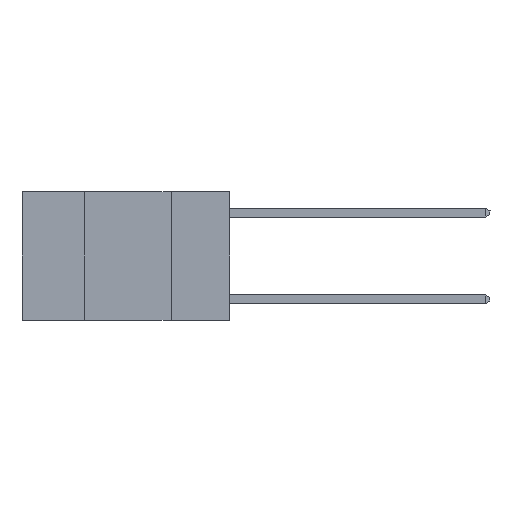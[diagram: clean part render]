
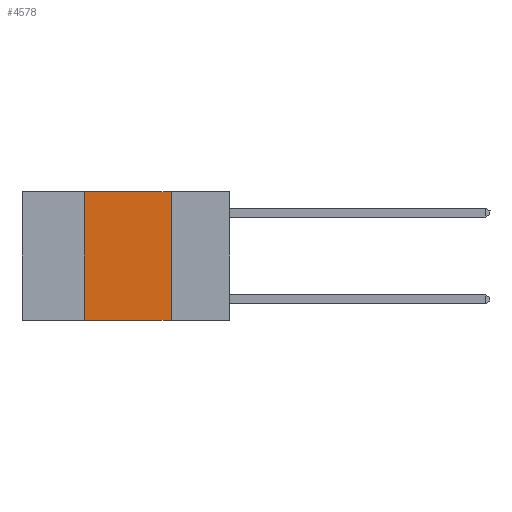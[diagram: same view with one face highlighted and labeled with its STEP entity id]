
A CAD part, left-side view. The second image highlights one B-rep face of the part: STEP entity #4578.
In plain terms, the highlighted planar face has unit normal (-1, 0, 0).
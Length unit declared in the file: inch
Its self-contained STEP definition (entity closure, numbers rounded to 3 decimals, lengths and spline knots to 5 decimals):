
#58 = VERTEX_POINT ( 'NONE', #2633 ) ;
#358 = VECTOR ( 'NONE', #4626, 39.37008 ) ;
#368 = CARTESIAN_POINT ( 'NONE',  ( 0., 0.42, -0.37 ) ) ;
#1398 = DIRECTION ( 'NONE',  ( 0., 0., 1. ) ) ;
#1654 = VECTOR ( 'NONE', #1398, 39.37008 ) ;
#1750 = EDGE_CURVE ( 'NONE', #11668, #8958, #3074, .T. ) ;
#1890 = VECTOR ( 'NONE', #10463, 39.37008 ) ;
#2633 = CARTESIAN_POINT ( 'NONE',  ( 0., 0.17, -0.37 ) ) ;
#2712 = PLANE ( 'NONE',  #10437 ) ;
#2893 = VERTEX_POINT ( 'NONE', #368 ) ;
#3074 = LINE ( 'NONE', #10550, #358 ) ;
#3284 = CARTESIAN_POINT ( 'NONE',  ( 0., 0.6, -0.37 ) ) ;
#3461 = LINE ( 'NONE', #3741, #5875 ) ;
#3641 = DIRECTION ( 'NONE',  ( 1., 0., 0. ) ) ;
#3741 = CARTESIAN_POINT ( 'NONE',  ( 0., 0.17, 0. ) ) ;
#4429 = ORIENTED_EDGE ( 'NONE', *, *, #9628, .T. ) ;
#4501 = CARTESIAN_POINT ( 'NONE',  ( 0., 0.6, 0. ) ) ;
#4578 = ADVANCED_FACE ( 'NONE', ( #8451 ), #2712, .F. ) ;
#4626 = DIRECTION ( 'NONE',  ( 0., -1., 0. ) ) ;
#5115 = CARTESIAN_POINT ( 'NONE',  ( 0., 0.17, 0. ) ) ;
#5264 = EDGE_CURVE ( 'NONE', #2893, #11668, #6473, .T. ) ;
#5408 = EDGE_LOOP ( 'NONE', ( #8092, #6256, #6558, #4429 ) ) ;
#5875 = VECTOR ( 'NONE', #10898, 39.37008 ) ;
#6256 = ORIENTED_EDGE ( 'NONE', *, *, #1750, .F. ) ;
#6473 = LINE ( 'NONE', #6831, #1654 ) ;
#6558 = ORIENTED_EDGE ( 'NONE', *, *, #5264, .F. ) ;
#6831 = CARTESIAN_POINT ( 'NONE',  ( 0., 0.42, 0. ) ) ;
#8092 = ORIENTED_EDGE ( 'NONE', *, *, #9266, .F. ) ;
#8451 = FACE_OUTER_BOUND ( 'NONE', #5408, .T. ) ;
#8958 = VERTEX_POINT ( 'NONE', #5115 ) ;
#9177 = CARTESIAN_POINT ( 'NONE',  ( 0., 0.42, 0. ) ) ;
#9266 = EDGE_CURVE ( 'NONE', #8958, #58, #3461, .T. ) ;
#9628 = EDGE_CURVE ( 'NONE', #2893, #58, #11436, .T. ) ;
#9905 = DIRECTION ( 'NONE',  ( 0., 0., -1. ) ) ;
#10437 = AXIS2_PLACEMENT_3D ( 'NONE', #4501, #3641, #9905 ) ;
#10463 = DIRECTION ( 'NONE',  ( 0., -1., 0. ) ) ;
#10550 = CARTESIAN_POINT ( 'NONE',  ( 0., 0.6, 0. ) ) ;
#10898 = DIRECTION ( 'NONE',  ( 0., 0., -1. ) ) ;
#11436 = LINE ( 'NONE', #3284, #1890 ) ;
#11668 = VERTEX_POINT ( 'NONE', #9177 ) ;
